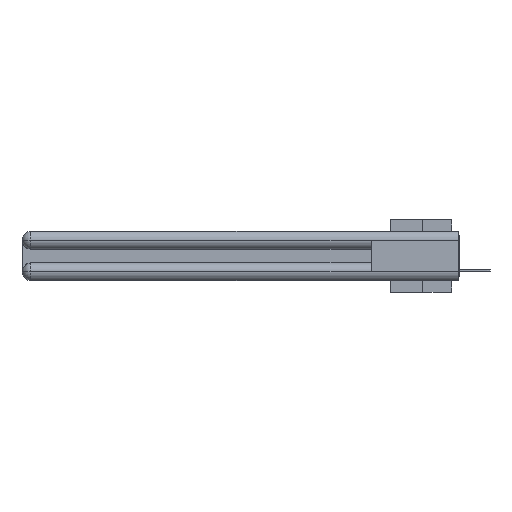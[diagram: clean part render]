
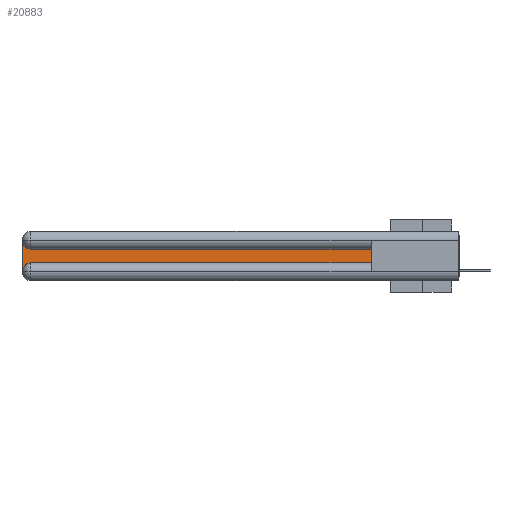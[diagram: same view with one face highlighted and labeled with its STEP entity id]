
A CAD part, left-side view. The second image highlights one B-rep face of the part: STEP entity #20883.
In plain terms, the highlighted planar face has unit normal (-1, 0, 0).
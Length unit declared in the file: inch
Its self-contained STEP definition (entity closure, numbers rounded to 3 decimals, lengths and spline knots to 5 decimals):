
#499 = DIRECTION ( 'NONE',  ( 1., 0., 0. ) ) ;
#920 = EDGE_CURVE ( 'NONE', #37203, #33985, #8648, .T. ) ;
#964 = CARTESIAN_POINT ( 'NONE',  ( 0.075, 0.6, -0.1225 ) ) ;
#1198 = CARTESIAN_POINT ( 'NONE',  ( 0.075, 0.6, -0.2175 ) ) ;
#1383 = CARTESIAN_POINT ( 'NONE',  ( 0.075, 0.6, -0.2175 ) ) ;
#2262 = ORIENTED_EDGE ( 'NONE', *, *, #16313, .T. ) ;
#2610 = EDGE_CURVE ( 'NONE', #30966, #37203, #27959, .T. ) ;
#3658 = VERTEX_POINT ( 'NONE', #1198 ) ;
#4295 = LINE ( 'NONE', #17490, #5685 ) ;
#4545 = EDGE_CURVE ( 'NONE', #24515, #30966, #22089, .T. ) ;
#5685 = VECTOR ( 'NONE', #38393, 39.37008 ) ;
#6288 = EDGE_CURVE ( 'NONE', #3658, #6621, #4295, .T. ) ;
#6514 = CARTESIAN_POINT ( 'NONE',  ( 0.075, 0.6, -0.1225 ) ) ;
#6621 = VERTEX_POINT ( 'NONE', #964 ) ;
#6871 = DIRECTION ( 'NONE',  ( 1., 0., 0. ) ) ;
#7653 = ORIENTED_EDGE ( 'NONE', *, *, #920, .T. ) ;
#8412 = CARTESIAN_POINT ( 'NONE',  ( 0.075, 3., -0.0625 ) ) ;
#8648 = CIRCLE ( 'NONE', #17116, 0.06 ) ;
#8712 = FACE_OUTER_BOUND ( 'NONE', #10923, .T. ) ;
#9916 = VECTOR ( 'NONE', #32430, 39.37008 ) ;
#10131 = ORIENTED_EDGE ( 'NONE', *, *, #4545, .T. ) ;
#10923 = EDGE_LOOP ( 'NONE', ( #38855, #10131, #17631, #7653, #2262, #34112 ) ) ;
#15165 = DIRECTION ( 'NONE',  ( 0., 0., -1. ) ) ;
#16313 = EDGE_CURVE ( 'NONE', #33985, #3658, #17598, .T. ) ;
#16552 = AXIS2_PLACEMENT_3D ( 'NONE', #22092, #6871, #19265 ) ;
#17086 = CARTESIAN_POINT ( 'NONE',  ( 0.075, 2.94, -0.0625 ) ) ;
#17116 = AXIS2_PLACEMENT_3D ( 'NONE', #27205, #18647, #37309 ) ;
#17490 = CARTESIAN_POINT ( 'NONE',  ( 0.075, 0.6, -0.2175 ) ) ;
#17598 = LINE ( 'NONE', #1383, #9916 ) ;
#17631 = ORIENTED_EDGE ( 'NONE', *, *, #2610, .T. ) ;
#18647 = DIRECTION ( 'NONE',  ( 1., 0., 0. ) ) ;
#19112 = DIRECTION ( 'NONE',  ( 0., 1., 0. ) ) ;
#19265 = DIRECTION ( 'NONE',  ( 0., 0., -1. ) ) ;
#19682 = CARTESIAN_POINT ( 'NONE',  ( 0.075, 2.94, -0.2175 ) ) ;
#19951 = VECTOR ( 'NONE', #15165, 39.37008 ) ;
#20883 = ADVANCED_FACE ( 'NONE', ( #8712 ), #34473, .F. ) ;
#22089 = CIRCLE ( 'NONE', #25331, 0.06 ) ;
#22092 = CARTESIAN_POINT ( 'NONE',  ( 0.075, 3., -0.1225 ) ) ;
#24319 = CARTESIAN_POINT ( 'NONE',  ( 0.075, 3., -0.2175 ) ) ;
#24515 = VERTEX_POINT ( 'NONE', #35582 ) ;
#25331 = AXIS2_PLACEMENT_3D ( 'NONE', #17086, #499, #34383 ) ;
#27205 = CARTESIAN_POINT ( 'NONE',  ( 0.075, 2.94, -0.2775 ) ) ;
#27959 = LINE ( 'NONE', #24319, #19951 ) ;
#29729 = CARTESIAN_POINT ( 'NONE',  ( 0.075, 3., -0.2775 ) ) ;
#30966 = VERTEX_POINT ( 'NONE', #8412 ) ;
#32430 = DIRECTION ( 'NONE',  ( 0., -1., 0. ) ) ;
#33537 = EDGE_CURVE ( 'NONE', #6621, #24515, #37769, .T. ) ;
#33985 = VERTEX_POINT ( 'NONE', #19682 ) ;
#34112 = ORIENTED_EDGE ( 'NONE', *, *, #6288, .T. ) ;
#34383 = DIRECTION ( 'NONE',  ( 0., 0., -1. ) ) ;
#34473 = PLANE ( 'NONE',  #16552 ) ;
#35582 = CARTESIAN_POINT ( 'NONE',  ( 0.075, 2.94, -0.1225 ) ) ;
#37203 = VERTEX_POINT ( 'NONE', #29729 ) ;
#37309 = DIRECTION ( 'NONE',  ( 0., 0., -1. ) ) ;
#37769 = LINE ( 'NONE', #6514, #39013 ) ;
#38393 = DIRECTION ( 'NONE',  ( 0., 0., 1. ) ) ;
#38855 = ORIENTED_EDGE ( 'NONE', *, *, #33537, .T. ) ;
#39013 = VECTOR ( 'NONE', #19112, 39.37008 ) ;
